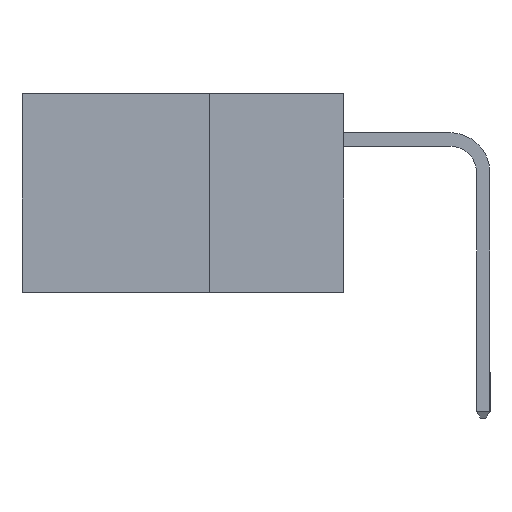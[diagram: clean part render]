
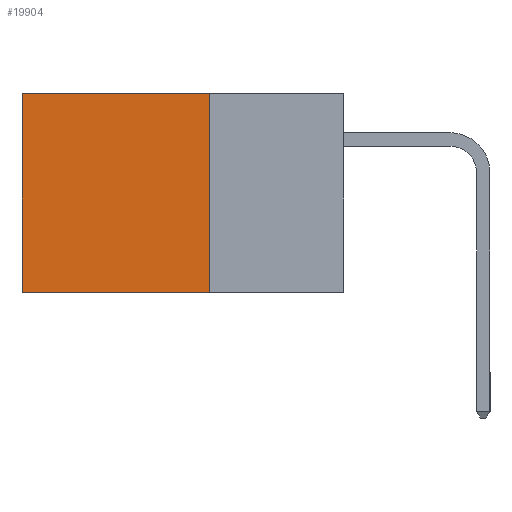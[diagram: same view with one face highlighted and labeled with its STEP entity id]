
A CAD part, left-side view. The second image highlights one B-rep face of the part: STEP entity #19904.
In plain terms, the highlighted planar face has unit normal (-1, 0, 0).
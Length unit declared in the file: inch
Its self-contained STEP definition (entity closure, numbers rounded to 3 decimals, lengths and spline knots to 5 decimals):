
#973 = PLANE ( 'NONE',  #10875 ) ;
#1837 = EDGE_LOOP ( 'NONE', ( #19375, #21858, #19387, #18192 ) ) ;
#3577 = EDGE_CURVE ( 'NONE', #13581, #20406, #9650, .T. ) ;
#4577 = EDGE_CURVE ( 'NONE', #19719, #20406, #5343, .T. ) ;
#5237 = VECTOR ( 'NONE', #14323, 39.37008 ) ;
#5343 = LINE ( 'NONE', #12309, #5237 ) ;
#5772 = LINE ( 'NONE', #16530, #8636 ) ;
#6440 = DIRECTION ( 'NONE',  ( 1., 0., 0. ) ) ;
#6562 = DIRECTION ( 'NONE',  ( 0., 0., -1. ) ) ;
#8636 = VECTOR ( 'NONE', #10867, 39.37008 ) ;
#9163 = VECTOR ( 'NONE', #20767, 39.37008 ) ;
#9205 = CARTESIAN_POINT ( 'NONE',  ( 0.2615, 0.25, -0.37 ) ) ;
#9498 = CARTESIAN_POINT ( 'NONE',  ( 0.2615, 0.6, 0. ) ) ;
#9650 = LINE ( 'NONE', #16999, #9163 ) ;
#10867 = DIRECTION ( 'NONE',  ( 0., 0., -1. ) ) ;
#10875 = AXIS2_PLACEMENT_3D ( 'NONE', #11993, #6440, #6562 ) ;
#11993 = CARTESIAN_POINT ( 'NONE',  ( 0.2615, 0.25, -0.37 ) ) ;
#12309 = CARTESIAN_POINT ( 'NONE',  ( 0.2615, 0.6, -0.37 ) ) ;
#13581 = VERTEX_POINT ( 'NONE', #9205 ) ;
#14323 = DIRECTION ( 'NONE',  ( 0., 0., -1. ) ) ;
#15449 = VERTEX_POINT ( 'NONE', #18591 ) ;
#15919 = LINE ( 'NONE', #23226, #16517 ) ;
#16035 = DIRECTION ( 'NONE',  ( 0., 1., 0. ) ) ;
#16517 = VECTOR ( 'NONE', #16035, 39.37008 ) ;
#16530 = CARTESIAN_POINT ( 'NONE',  ( 0.2615, 0.25, -0.37 ) ) ;
#16999 = CARTESIAN_POINT ( 'NONE',  ( 0.2615, 0.25, -0.37 ) ) ;
#17188 = FACE_OUTER_BOUND ( 'NONE', #1837, .T. ) ;
#18192 = ORIENTED_EDGE ( 'NONE', *, *, #19966, .T. ) ;
#18591 = CARTESIAN_POINT ( 'NONE',  ( 0.2615, 0.25, 0. ) ) ;
#19375 = ORIENTED_EDGE ( 'NONE', *, *, #4577, .T. ) ;
#19387 = ORIENTED_EDGE ( 'NONE', *, *, #20969, .F. ) ;
#19719 = VERTEX_POINT ( 'NONE', #9498 ) ;
#19904 = ADVANCED_FACE ( 'NONE', ( #17188 ), #973, .F. ) ;
#19966 = EDGE_CURVE ( 'NONE', #15449, #19719, #15919, .T. ) ;
#20406 = VERTEX_POINT ( 'NONE', #21548 ) ;
#20767 = DIRECTION ( 'NONE',  ( 0., 1., 0. ) ) ;
#20969 = EDGE_CURVE ( 'NONE', #15449, #13581, #5772, .T. ) ;
#21548 = CARTESIAN_POINT ( 'NONE',  ( 0.2615, 0.6, -0.37 ) ) ;
#21858 = ORIENTED_EDGE ( 'NONE', *, *, #3577, .F. ) ;
#23226 = CARTESIAN_POINT ( 'NONE',  ( 0.2615, 0.25, 0. ) ) ;
